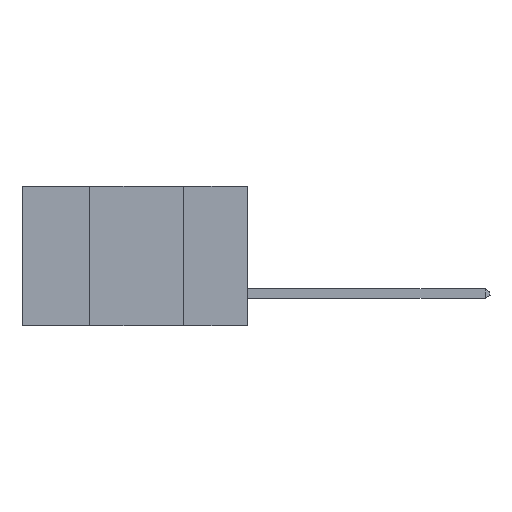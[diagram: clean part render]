
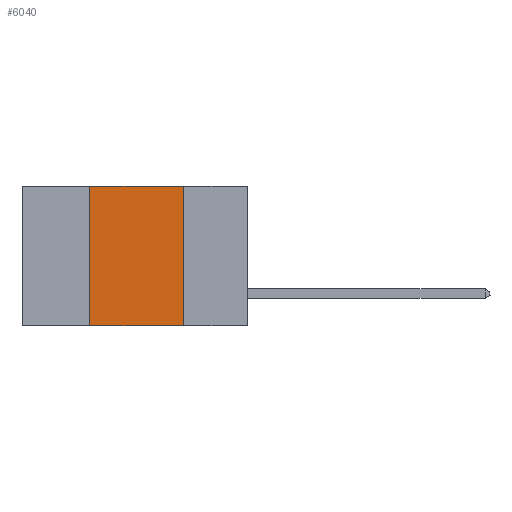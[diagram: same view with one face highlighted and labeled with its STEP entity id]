
A CAD part, left-side view. The second image highlights one B-rep face of the part: STEP entity #6040.
In plain terms, the highlighted planar face has unit normal (-1, 0, 0).
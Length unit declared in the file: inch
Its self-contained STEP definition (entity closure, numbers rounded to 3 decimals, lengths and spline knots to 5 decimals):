
#297 = DIRECTION ( 'NONE',  ( 0., 0., -1. ) ) ;
#320 = VERTEX_POINT ( 'NONE', #5577 ) ;
#616 = CARTESIAN_POINT ( 'NONE',  ( 0., 0.6, 0. ) ) ;
#1440 = EDGE_CURVE ( 'NONE', #10719, #7019, #11978, .T. ) ;
#1880 = DIRECTION ( 'NONE',  ( 0., 0., 1. ) ) ;
#1999 = LINE ( 'NONE', #14575, #10712 ) ;
#2553 = VECTOR ( 'NONE', #297, 39.37008 ) ;
#2676 = DIRECTION ( 'NONE',  ( 0., -1., 0. ) ) ;
#3498 = VECTOR ( 'NONE', #1880, 39.37008 ) ;
#3630 = EDGE_CURVE ( 'NONE', #13934, #7019, #4610, .T. ) ;
#3785 = CARTESIAN_POINT ( 'NONE',  ( 0., 0.6, -0.37 ) ) ;
#4141 = DIRECTION ( 'NONE',  ( 0., 0., -1. ) ) ;
#4610 = LINE ( 'NONE', #3785, #13330 ) ;
#5183 = EDGE_CURVE ( 'NONE', #13934, #320, #7060, .T. ) ;
#5196 = CARTESIAN_POINT ( 'NONE',  ( 0., 0.42, 0. ) ) ;
#5400 = FACE_OUTER_BOUND ( 'NONE', #5590, .T. ) ;
#5577 = CARTESIAN_POINT ( 'NONE',  ( 0., 0.42, 0. ) ) ;
#5590 = EDGE_LOOP ( 'NONE', ( #11665, #11289, #7634, #6102 ) ) ;
#6040 = ADVANCED_FACE ( 'NONE', ( #5400 ), #10785, .F. ) ;
#6102 = ORIENTED_EDGE ( 'NONE', *, *, #3630, .T. ) ;
#7019 = VERTEX_POINT ( 'NONE', #8215 ) ;
#7060 = LINE ( 'NONE', #5196, #3498 ) ;
#7634 = ORIENTED_EDGE ( 'NONE', *, *, #5183, .F. ) ;
#7745 = DIRECTION ( 'NONE',  ( 0., -1., 0. ) ) ;
#8215 = CARTESIAN_POINT ( 'NONE',  ( 0., 0.17, -0.37 ) ) ;
#9028 = CARTESIAN_POINT ( 'NONE',  ( 0., 0.17, 0. ) ) ;
#9386 = CARTESIAN_POINT ( 'NONE',  ( 0., 0.42, -0.37 ) ) ;
#10712 = VECTOR ( 'NONE', #7745, 39.37008 ) ;
#10719 = VERTEX_POINT ( 'NONE', #14570 ) ;
#10785 = PLANE ( 'NONE',  #14467 ) ;
#11289 = ORIENTED_EDGE ( 'NONE', *, *, #13525, .F. ) ;
#11665 = ORIENTED_EDGE ( 'NONE', *, *, #1440, .F. ) ;
#11978 = LINE ( 'NONE', #9028, #2553 ) ;
#12032 = DIRECTION ( 'NONE',  ( 1., 0., 0. ) ) ;
#13330 = VECTOR ( 'NONE', #2676, 39.37008 ) ;
#13525 = EDGE_CURVE ( 'NONE', #320, #10719, #1999, .T. ) ;
#13934 = VERTEX_POINT ( 'NONE', #9386 ) ;
#14467 = AXIS2_PLACEMENT_3D ( 'NONE', #616, #12032, #4141 ) ;
#14570 = CARTESIAN_POINT ( 'NONE',  ( 0., 0.17, 0. ) ) ;
#14575 = CARTESIAN_POINT ( 'NONE',  ( 0., 0.6, 0. ) ) ;
